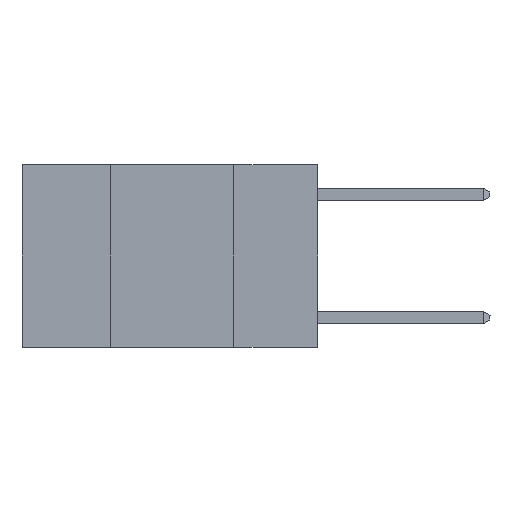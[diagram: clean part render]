
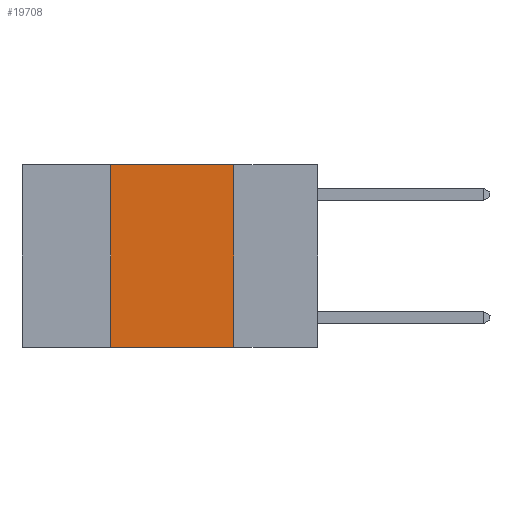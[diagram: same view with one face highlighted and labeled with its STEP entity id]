
A CAD part, left-side view. The second image highlights one B-rep face of the part: STEP entity #19708.
In plain terms, the highlighted planar face has unit normal (-1, 0, 0).
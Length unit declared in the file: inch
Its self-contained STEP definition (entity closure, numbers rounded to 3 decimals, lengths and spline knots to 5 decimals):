
#811 = ORIENTED_EDGE ( 'NONE', *, *, #26713, .F. ) ;
#1295 = VECTOR ( 'NONE', #11320, 39.37008 ) ;
#1513 = CARTESIAN_POINT ( 'NONE',  ( 0., 0.6, 0. ) ) ;
#2172 = VECTOR ( 'NONE', #25935, 39.37008 ) ;
#2240 = EDGE_CURVE ( 'NONE', #4018, #20428, #26052, .T. ) ;
#2394 = LINE ( 'NONE', #13652, #14655 ) ;
#2603 = FACE_OUTER_BOUND ( 'NONE', #9932, .T. ) ;
#3376 = CARTESIAN_POINT ( 'NONE',  ( 0., 0.17, -0.37 ) ) ;
#4018 = VERTEX_POINT ( 'NONE', #23039 ) ;
#6368 = AXIS2_PLACEMENT_3D ( 'NONE', #20625, #27180, #14100 ) ;
#6670 = ORIENTED_EDGE ( 'NONE', *, *, #7291, .T. ) ;
#7291 = EDGE_CURVE ( 'NONE', #8301, #22410, #22356, .T. ) ;
#8301 = VERTEX_POINT ( 'NONE', #22128 ) ;
#9932 = EDGE_LOOP ( 'NONE', ( #27783, #11137, #811, #6670 ) ) ;
#11137 = ORIENTED_EDGE ( 'NONE', *, *, #2240, .F. ) ;
#11320 = DIRECTION ( 'NONE',  ( 0., 0., 1. ) ) ;
#13652 = CARTESIAN_POINT ( 'NONE',  ( 0., 0.17, 0. ) ) ;
#14100 = DIRECTION ( 'NONE',  ( 0., 0., -1. ) ) ;
#14655 = VECTOR ( 'NONE', #26708, 39.37008 ) ;
#19708 = ADVANCED_FACE ( 'NONE', ( #2603 ), #25017, .F. ) ;
#20221 = CARTESIAN_POINT ( 'NONE',  ( 0., 0.6, -0.37 ) ) ;
#20428 = VERTEX_POINT ( 'NONE', #27147 ) ;
#20625 = CARTESIAN_POINT ( 'NONE',  ( 0., 0.6, 0. ) ) ;
#22128 = CARTESIAN_POINT ( 'NONE',  ( 0., 0.42, -0.37 ) ) ;
#22197 = CARTESIAN_POINT ( 'NONE',  ( 0., 0.42, 0. ) ) ;
#22356 = LINE ( 'NONE', #20221, #23032 ) ;
#22410 = VERTEX_POINT ( 'NONE', #3376 ) ;
#22446 = DIRECTION ( 'NONE',  ( 0., -1., 0. ) ) ;
#22876 = EDGE_CURVE ( 'NONE', #20428, #22410, #2394, .T. ) ;
#23032 = VECTOR ( 'NONE', #22446, 39.37008 ) ;
#23039 = CARTESIAN_POINT ( 'NONE',  ( 0., 0.42, 0. ) ) ;
#23876 = LINE ( 'NONE', #22197, #1295 ) ;
#25017 = PLANE ( 'NONE',  #6368 ) ;
#25935 = DIRECTION ( 'NONE',  ( 0., -1., 0. ) ) ;
#26052 = LINE ( 'NONE', #1513, #2172 ) ;
#26708 = DIRECTION ( 'NONE',  ( 0., 0., -1. ) ) ;
#26713 = EDGE_CURVE ( 'NONE', #8301, #4018, #23876, .T. ) ;
#27147 = CARTESIAN_POINT ( 'NONE',  ( 0., 0.17, 0. ) ) ;
#27180 = DIRECTION ( 'NONE',  ( 1., 0., 0. ) ) ;
#27783 = ORIENTED_EDGE ( 'NONE', *, *, #22876, .F. ) ;
